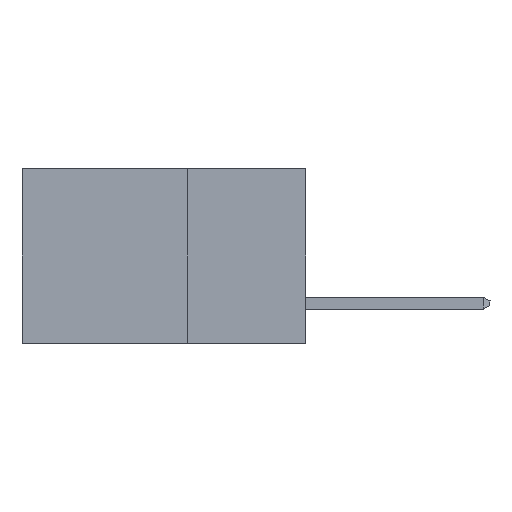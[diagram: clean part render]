
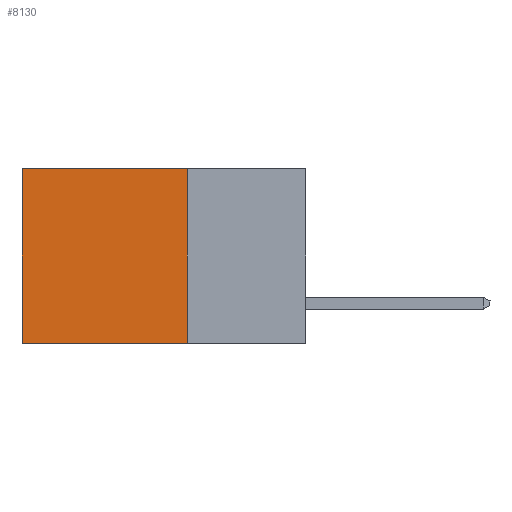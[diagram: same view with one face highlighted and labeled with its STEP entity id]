
A CAD part, left-side view. The second image highlights one B-rep face of the part: STEP entity #8130.
In plain terms, the highlighted planar face has unit normal (-1, 0, 0).
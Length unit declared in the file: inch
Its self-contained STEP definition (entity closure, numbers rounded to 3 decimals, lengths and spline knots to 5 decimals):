
#169 = LINE ( 'NONE', #21319, #23231 ) ;
#283 = EDGE_LOOP ( 'NONE', ( #826, #7785, #9575, #568 ) ) ;
#568 = ORIENTED_EDGE ( 'NONE', *, *, #18049, .T. ) ;
#686 = CARTESIAN_POINT ( 'NONE',  ( 0.298, 0.25, -0.37 ) ) ;
#826 = ORIENTED_EDGE ( 'NONE', *, *, #17190, .T. ) ;
#1199 = DIRECTION ( 'NONE',  ( 0., 1., 0. ) ) ;
#1668 = CARTESIAN_POINT ( 'NONE',  ( 0.298, 0.25, -0.37 ) ) ;
#1737 = DIRECTION ( 'NONE',  ( 1., 0., 0. ) ) ;
#2078 = DIRECTION ( 'NONE',  ( 0., 0., -1. ) ) ;
#3123 = CARTESIAN_POINT ( 'NONE',  ( 0.298, 0.25, 0. ) ) ;
#3584 = DIRECTION ( 'NONE',  ( 0., 0., -1. ) ) ;
#5394 = DIRECTION ( 'NONE',  ( 0., 0., -1. ) ) ;
#6049 = VECTOR ( 'NONE', #16474, 39.37008 ) ;
#6246 = VECTOR ( 'NONE', #1199, 39.37008 ) ;
#6938 = EDGE_CURVE ( 'NONE', #18352, #17476, #21627, .T. ) ;
#7785 = ORIENTED_EDGE ( 'NONE', *, *, #6938, .F. ) ;
#7901 = VERTEX_POINT ( 'NONE', #19068 ) ;
#8130 = ADVANCED_FACE ( 'NONE', ( #13511 ), #21793, .F. ) ;
#9359 = VERTEX_POINT ( 'NONE', #14870 ) ;
#9575 = ORIENTED_EDGE ( 'NONE', *, *, #14897, .F. ) ;
#9708 = VECTOR ( 'NONE', #2078, 39.37008 ) ;
#12363 = CARTESIAN_POINT ( 'NONE',  ( 0.298, 0.6, -0.37 ) ) ;
#13432 = CARTESIAN_POINT ( 'NONE',  ( 0.298, 0.6, 0. ) ) ;
#13511 = FACE_OUTER_BOUND ( 'NONE', #283, .T. ) ;
#14267 = AXIS2_PLACEMENT_3D ( 'NONE', #23765, #1737, #3584 ) ;
#14870 = CARTESIAN_POINT ( 'NONE',  ( 0.298, 0.6, 0. ) ) ;
#14897 = EDGE_CURVE ( 'NONE', #7901, #18352, #169, .T. ) ;
#16474 = DIRECTION ( 'NONE',  ( 0., 1., 0. ) ) ;
#16889 = LINE ( 'NONE', #3123, #6246 ) ;
#17190 = EDGE_CURVE ( 'NONE', #9359, #17476, #21555, .T. ) ;
#17476 = VERTEX_POINT ( 'NONE', #12363 ) ;
#18049 = EDGE_CURVE ( 'NONE', #7901, #9359, #16889, .T. ) ;
#18352 = VERTEX_POINT ( 'NONE', #686 ) ;
#19068 = CARTESIAN_POINT ( 'NONE',  ( 0.298, 0.25, 0. ) ) ;
#21319 = CARTESIAN_POINT ( 'NONE',  ( 0.298, 0.25, 0. ) ) ;
#21555 = LINE ( 'NONE', #13432, #9708 ) ;
#21627 = LINE ( 'NONE', #1668, #6049 ) ;
#21793 = PLANE ( 'NONE',  #14267 ) ;
#23231 = VECTOR ( 'NONE', #5394, 39.37008 ) ;
#23765 = CARTESIAN_POINT ( 'NONE',  ( 0.298, 0.25, 0. ) ) ;
